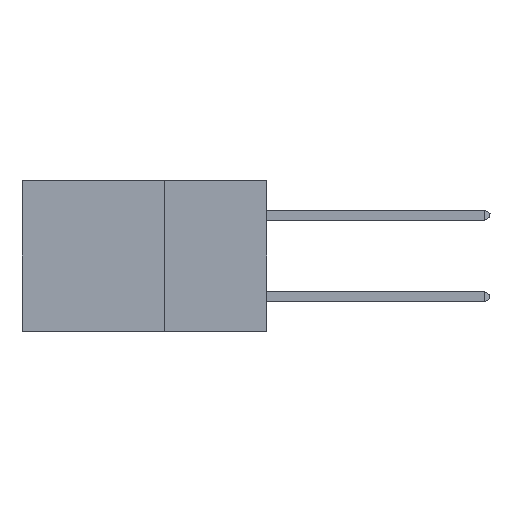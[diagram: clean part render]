
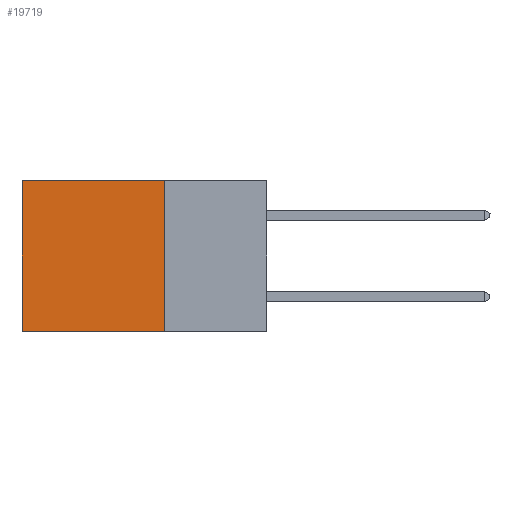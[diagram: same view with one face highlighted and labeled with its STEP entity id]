
A CAD part, left-side view. The second image highlights one B-rep face of the part: STEP entity #19719.
In plain terms, the highlighted planar face has unit normal (-1, 0, 0).
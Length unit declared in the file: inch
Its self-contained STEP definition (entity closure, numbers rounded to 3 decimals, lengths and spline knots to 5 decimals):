
#712 = DIRECTION ( 'NONE',  ( 0., 1., 0. ) ) ;
#811 = ORIENTED_EDGE ( 'NONE', *, *, #21654, .F. ) ;
#908 = CARTESIAN_POINT ( 'NONE',  ( 0.2875, 0.25, -0.37 ) ) ;
#1119 = LINE ( 'NONE', #28201, #4424 ) ;
#3117 = CARTESIAN_POINT ( 'NONE',  ( 0.2875, 0.25, 0. ) ) ;
#4051 = AXIS2_PLACEMENT_3D ( 'NONE', #27591, #29974, #27913 ) ;
#4424 = VECTOR ( 'NONE', #30586, 39.37008 ) ;
#4597 = CARTESIAN_POINT ( 'NONE',  ( 0.2875, 0.6, 0. ) ) ;
#6646 = CARTESIAN_POINT ( 'NONE',  ( 0.2875, 0.25, 0. ) ) ;
#6836 = DIRECTION ( 'NONE',  ( 0., 0., -1. ) ) ;
#6909 = ORIENTED_EDGE ( 'NONE', *, *, #14631, .F. ) ;
#8305 = FACE_OUTER_BOUND ( 'NONE', #25715, .T. ) ;
#8328 = ORIENTED_EDGE ( 'NONE', *, *, #28372, .T. ) ;
#8946 = VECTOR ( 'NONE', #712, 39.37008 ) ;
#9226 = CARTESIAN_POINT ( 'NONE',  ( 0.2875, 0.25, 0. ) ) ;
#12476 = VERTEX_POINT ( 'NONE', #15715 ) ;
#12976 = VECTOR ( 'NONE', #14554, 39.37008 ) ;
#14554 = DIRECTION ( 'NONE',  ( 0., 0., -1. ) ) ;
#14631 = EDGE_CURVE ( 'NONE', #20574, #12476, #1119, .T. ) ;
#15075 = LINE ( 'NONE', #3117, #8946 ) ;
#15715 = CARTESIAN_POINT ( 'NONE',  ( 0.2875, 0.6, -0.37 ) ) ;
#16472 = VERTEX_POINT ( 'NONE', #6646 ) ;
#18923 = VECTOR ( 'NONE', #6836, 39.37008 ) ;
#19719 = ADVANCED_FACE ( 'NONE', ( #8305 ), #20592, .F. ) ;
#20574 = VERTEX_POINT ( 'NONE', #908 ) ;
#20592 = PLANE ( 'NONE',  #4051 ) ;
#21078 = ORIENTED_EDGE ( 'NONE', *, *, #29617, .T. ) ;
#21525 = VERTEX_POINT ( 'NONE', #4597 ) ;
#21654 = EDGE_CURVE ( 'NONE', #16472, #20574, #31035, .T. ) ;
#23795 = LINE ( 'NONE', #26813, #12976 ) ;
#25715 = EDGE_LOOP ( 'NONE', ( #8328, #6909, #811, #21078 ) ) ;
#26813 = CARTESIAN_POINT ( 'NONE',  ( 0.2875, 0.6, 0. ) ) ;
#27591 = CARTESIAN_POINT ( 'NONE',  ( 0.2875, 0.25, 0. ) ) ;
#27913 = DIRECTION ( 'NONE',  ( 0., 0., -1. ) ) ;
#28201 = CARTESIAN_POINT ( 'NONE',  ( 0.2875, 0.25, -0.37 ) ) ;
#28372 = EDGE_CURVE ( 'NONE', #21525, #12476, #23795, .T. ) ;
#29617 = EDGE_CURVE ( 'NONE', #16472, #21525, #15075, .T. ) ;
#29974 = DIRECTION ( 'NONE',  ( 1., 0., 0. ) ) ;
#30586 = DIRECTION ( 'NONE',  ( 0., 1., 0. ) ) ;
#31035 = LINE ( 'NONE', #9226, #18923 ) ;
